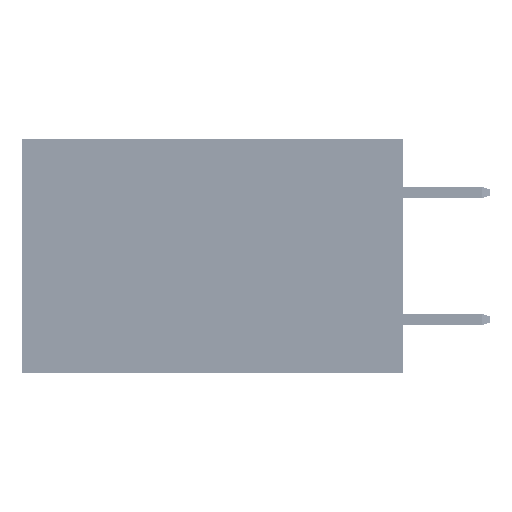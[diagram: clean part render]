
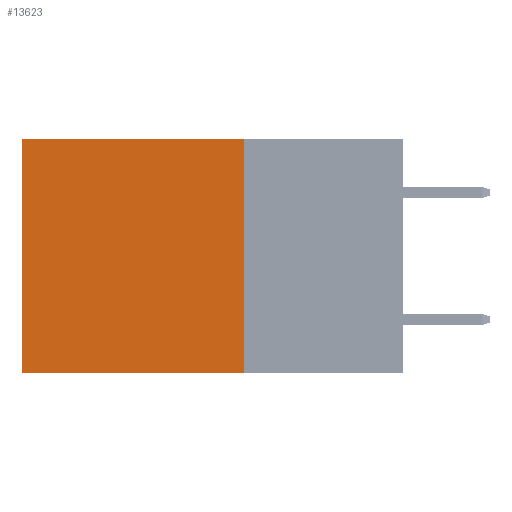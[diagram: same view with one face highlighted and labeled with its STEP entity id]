
A CAD part, left-side view. The second image highlights one B-rep face of the part: STEP entity #13623.
In plain terms, the highlighted planar face has unit normal (-1, 0, 0).
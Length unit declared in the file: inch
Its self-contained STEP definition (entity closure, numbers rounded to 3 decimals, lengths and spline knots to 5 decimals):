
#458 = VERTEX_POINT ( 'NONE', #16506 ) ;
#758 = CARTESIAN_POINT ( 'NONE',  ( 0.2875, 0.25, -0.37 ) ) ;
#1175 = CARTESIAN_POINT ( 'NONE',  ( 0.2875, 0.25, 0. ) ) ;
#1664 = DIRECTION ( 'NONE',  ( 1., 0., 0. ) ) ;
#2000 = VECTOR ( 'NONE', #17735, 39.37008 ) ;
#2807 = CARTESIAN_POINT ( 'NONE',  ( 0.2875, 0.6, 0. ) ) ;
#2852 = EDGE_CURVE ( 'NONE', #38512, #11231, #40588, .T. ) ;
#5704 = LINE ( 'NONE', #45945, #9920 ) ;
#6552 = CARTESIAN_POINT ( 'NONE',  ( 0.2875, 0.25, -0.37 ) ) ;
#7127 = DIRECTION ( 'NONE',  ( 0., 1., 0. ) ) ;
#8847 = ORIENTED_EDGE ( 'NONE', *, *, #18906, .T. ) ;
#9920 = VECTOR ( 'NONE', #12278, 39.37008 ) ;
#10430 = EDGE_CURVE ( 'NONE', #31227, #458, #32297, .T. ) ;
#11231 = VERTEX_POINT ( 'NONE', #2807 ) ;
#11584 = CARTESIAN_POINT ( 'NONE',  ( 0.2875, 0.25, 0. ) ) ;
#12278 = DIRECTION ( 'NONE',  ( 0., 0., -1. ) ) ;
#12684 = EDGE_CURVE ( 'NONE', #38512, #31227, #5704, .T. ) ;
#13623 = ADVANCED_FACE ( 'NONE', ( #20839 ), #46255, .F. ) ;
#15092 = EDGE_LOOP ( 'NONE', ( #8847, #26278, #19971, #30610 ) ) ;
#15512 = LINE ( 'NONE', #45050, #43516 ) ;
#15986 = DIRECTION ( 'NONE',  ( 0., 0., -1. ) ) ;
#16506 = CARTESIAN_POINT ( 'NONE',  ( 0.2875, 0.6, -0.37 ) ) ;
#17735 = DIRECTION ( 'NONE',  ( 0., 1., 0. ) ) ;
#17924 = VECTOR ( 'NONE', #7127, 39.37008 ) ;
#18906 = EDGE_CURVE ( 'NONE', #11231, #458, #15512, .T. ) ;
#19971 = ORIENTED_EDGE ( 'NONE', *, *, #12684, .F. ) ;
#20839 = FACE_OUTER_BOUND ( 'NONE', #15092, .T. ) ;
#25459 = AXIS2_PLACEMENT_3D ( 'NONE', #1175, #1664, #15986 ) ;
#26278 = ORIENTED_EDGE ( 'NONE', *, *, #10430, .F. ) ;
#29592 = DIRECTION ( 'NONE',  ( 0., 0., -1. ) ) ;
#30610 = ORIENTED_EDGE ( 'NONE', *, *, #2852, .T. ) ;
#31227 = VERTEX_POINT ( 'NONE', #758 ) ;
#32297 = LINE ( 'NONE', #6552, #2000 ) ;
#38512 = VERTEX_POINT ( 'NONE', #11584 ) ;
#40357 = CARTESIAN_POINT ( 'NONE',  ( 0.2875, 0.25, 0. ) ) ;
#40588 = LINE ( 'NONE', #40357, #17924 ) ;
#43516 = VECTOR ( 'NONE', #29592, 39.37008 ) ;
#45050 = CARTESIAN_POINT ( 'NONE',  ( 0.2875, 0.6, 0. ) ) ;
#45945 = CARTESIAN_POINT ( 'NONE',  ( 0.2875, 0.25, 0. ) ) ;
#46255 = PLANE ( 'NONE',  #25459 ) ;
